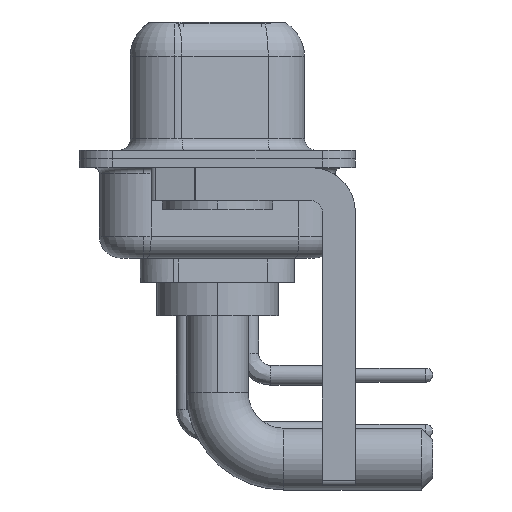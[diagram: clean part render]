
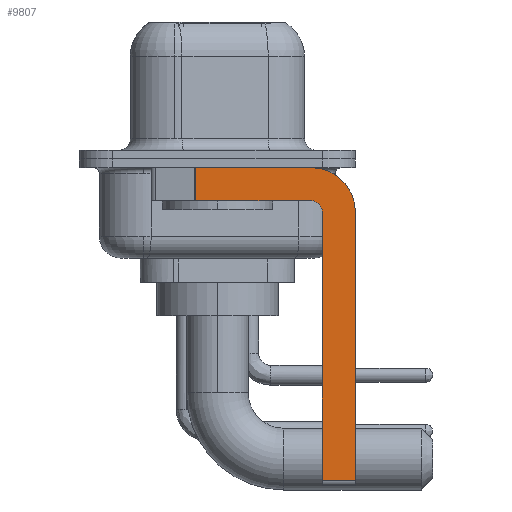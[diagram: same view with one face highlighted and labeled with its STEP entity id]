
A CAD part, left-side view. The second image highlights one B-rep face of the part: STEP entity #9807.
In plain terms, the highlighted planar face has unit normal (-1, 0, 0).
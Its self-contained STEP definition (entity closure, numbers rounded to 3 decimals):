
#339 = CARTESIAN_POINT ( 'NONE',  ( -2.9, -4.25, -1.9 ) ) ;
#562 = VECTOR ( 'NONE', #15430, 1000. ) ;
#631 = DIRECTION ( 'NONE',  ( 0., 1., 0. ) ) ;
#676 = VECTOR ( 'NONE', #5311, 1000. ) ;
#894 = EDGE_CURVE ( 'NONE', #10644, #9081, #3129, .T. ) ;
#955 = CARTESIAN_POINT ( 'NONE',  ( -2.9, -6.25, -2.4 ) ) ;
#1188 = ORIENTED_EDGE ( 'NONE', *, *, #17759, .F. ) ;
#1274 = EDGE_CURVE ( 'NONE', #11187, #5289, #12027, .T. ) ;
#1475 = CARTESIAN_POINT ( 'NONE',  ( -2.9, -4.25, -2.4 ) ) ;
#1975 = DIRECTION ( 'NONE',  ( 0., 0., -1. ) ) ;
#2250 = VERTEX_POINT ( 'NONE', #12343 ) ;
#2714 = VERTEX_POINT ( 'NONE', #16964 ) ;
#2839 = AXIS2_PLACEMENT_3D ( 'NONE', #1475, #4582, #1975 ) ;
#3129 = LINE ( 'NONE', #6241, #13294 ) ;
#4101 = CIRCLE ( 'NONE', #2839, 2. ) ;
#4295 = CARTESIAN_POINT ( 'NONE',  ( -2.9, 0.978, -1.9 ) ) ;
#4369 = CARTESIAN_POINT ( 'NONE',  ( -2.9, -6.25, -14.55 ) ) ;
#4582 = DIRECTION ( 'NONE',  ( 1., 0., 0. ) ) ;
#4643 = CARTESIAN_POINT ( 'NONE',  ( -2.9, -4.25, -2.4 ) ) ;
#4733 = DIRECTION ( 'NONE',  ( 0., -1., 0. ) ) ;
#4897 = AXIS2_PLACEMENT_3D ( 'NONE', #4643, #11170, #14164 ) ;
#5289 = VERTEX_POINT ( 'NONE', #4369 ) ;
#5295 = ORIENTED_EDGE ( 'NONE', *, *, #894, .F. ) ;
#5311 = DIRECTION ( 'NONE',  ( 0., 0., 1. ) ) ;
#5413 = CARTESIAN_POINT ( 'NONE',  ( -2.9, -4.75, -14.8 ) ) ;
#5931 = PLANE ( 'NONE',  #14846 ) ;
#6241 = CARTESIAN_POINT ( 'NONE',  ( -2.9, 3., -0.4 ) ) ;
#6264 = EDGE_CURVE ( 'NONE', #10644, #2714, #9109, .T. ) ;
#6425 = DIRECTION ( 'NONE',  ( 0., -1., 0. ) ) ;
#7205 = EDGE_CURVE ( 'NONE', #17281, #14496, #14493, .T. ) ;
#7308 = VECTOR ( 'NONE', #631, 1000. ) ;
#7344 = DIRECTION ( 'NONE',  ( 0., 0., -1. ) ) ;
#8311 = CARTESIAN_POINT ( 'NONE',  ( -2.9, -4.75, -2.4 ) ) ;
#8355 = EDGE_LOOP ( 'NONE', ( #5295, #14135, #19073, #18147, #10499, #17591, #1188, #15968 ) ) ;
#8665 = DIRECTION ( 'NONE',  ( 0., 0., -1. ) ) ;
#9081 = VERTEX_POINT ( 'NONE', #11288 ) ;
#9109 = LINE ( 'NONE', #4295, #562 ) ;
#9807 = ADVANCED_FACE ( 'NONE', ( #19671 ), #5931, .F. ) ;
#10499 = ORIENTED_EDGE ( 'NONE', *, *, #16766, .F. ) ;
#10644 = VERTEX_POINT ( 'NONE', #14887 ) ;
#11170 = DIRECTION ( 'NONE',  ( -1., 0., 0. ) ) ;
#11187 = VERTEX_POINT ( 'NONE', #11252 ) ;
#11252 = CARTESIAN_POINT ( 'NONE',  ( -2.9, -4.75, -14.55 ) ) ;
#11288 = CARTESIAN_POINT ( 'NONE',  ( -2.9, -4.25, -0.4 ) ) ;
#12027 = LINE ( 'NONE', #18158, #17536 ) ;
#12237 = CARTESIAN_POINT ( 'NONE',  ( -2.9, -4.25, -1.9 ) ) ;
#12343 = CARTESIAN_POINT ( 'NONE',  ( -2.9, -6.25, -2.4 ) ) ;
#12929 = LINE ( 'NONE', #5413, #676 ) ;
#13294 = VECTOR ( 'NONE', #4733, 1000. ) ;
#13596 = EDGE_CURVE ( 'NONE', #9081, #2250, #4101, .T. ) ;
#13824 = VECTOR ( 'NONE', #8665, 1000. ) ;
#14135 = ORIENTED_EDGE ( 'NONE', *, *, #6264, .T. ) ;
#14164 = DIRECTION ( 'NONE',  ( 0., 0., 1. ) ) ;
#14339 = LINE ( 'NONE', #339, #7308 ) ;
#14493 = CIRCLE ( 'NONE', #4897, 0.5 ) ;
#14496 = VERTEX_POINT ( 'NONE', #12237 ) ;
#14779 = LINE ( 'NONE', #955, #13824 ) ;
#14846 = AXIS2_PLACEMENT_3D ( 'NONE', #18176, #19772, #7344 ) ;
#14887 = CARTESIAN_POINT ( 'NONE',  ( -2.9, 0.978, -0.4 ) ) ;
#15430 = DIRECTION ( 'NONE',  ( 0., 0., -1. ) ) ;
#15968 = ORIENTED_EDGE ( 'NONE', *, *, #13596, .F. ) ;
#16766 = EDGE_CURVE ( 'NONE', #11187, #17281, #12929, .T. ) ;
#16964 = CARTESIAN_POINT ( 'NONE',  ( -2.9, 0.978, -1.9 ) ) ;
#17281 = VERTEX_POINT ( 'NONE', #8311 ) ;
#17536 = VECTOR ( 'NONE', #6425, 1000. ) ;
#17591 = ORIENTED_EDGE ( 'NONE', *, *, #1274, .T. ) ;
#17759 = EDGE_CURVE ( 'NONE', #2250, #5289, #14779, .T. ) ;
#18147 = ORIENTED_EDGE ( 'NONE', *, *, #7205, .F. ) ;
#18158 = CARTESIAN_POINT ( 'NONE',  ( -2.9, -4.25, -14.55 ) ) ;
#18176 = CARTESIAN_POINT ( 'NONE',  ( -2.9, -4.25, -2.4 ) ) ;
#19073 = ORIENTED_EDGE ( 'NONE', *, *, #19752, .F. ) ;
#19671 = FACE_OUTER_BOUND ( 'NONE', #8355, .T. ) ;
#19752 = EDGE_CURVE ( 'NONE', #14496, #2714, #14339, .T. ) ;
#19772 = DIRECTION ( 'NONE',  ( 1., 0., 0. ) ) ;
